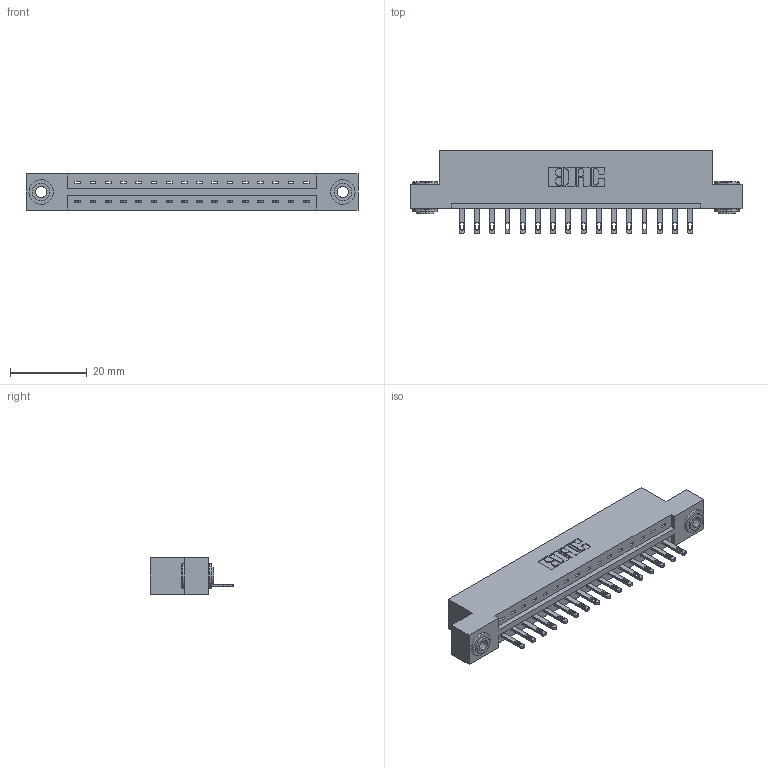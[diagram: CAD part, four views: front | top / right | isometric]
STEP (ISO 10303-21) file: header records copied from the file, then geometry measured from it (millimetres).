
FILE_DESCRIPTION (( 'STEP AP203' ), '1' );
FILE_NAME ('887-016-500-103.STEP', '2020-09-20T17:08:39', ( '' ), ( '' ), 'SwSTEP 2.0', 'SolidWorks 2020', '' );
FILE_SCHEMA (( 'CONFIG_CONTROL_DESIGN' ));
Length unit declared in the file: inch
Products named in the file (4): 887-016-500-103; 345-292-001_345-293-100; 837 Part_Flush Mounting Lugs - 0.156 Dia-TH; 345-250-002_345-250-002-102
Assembly tree (19 placements, depth 2):
  887-016-500-103
    837 Part_Flush Mounting Lugs - 0.156 Dia-TH
    345-292-001_345-293-100  x16
    345-250-002_345-250-002-102  x2
Bounding box: 86.41 x 21.85 x 9.4 mm (x, y, z)
Volume: 8684.9 mm3; surface area: 9100.3 mm2
Topology: 19 solids, 19 shells, 1080 faces, 3267 edges, 2174 vertices
Faces by surface type: plane 720, cylinder 352, cone 8
Entity records: 15836 total; most frequent: CARTESIAN_POINT 2733, ORIENTED_EDGE 2678, DIRECTION 2389, EDGE_CURVE 1339, VECTOR 1183, LINE 1183, VERTEX_POINT 890, AXIS2_PLACEMENT_3D 603
